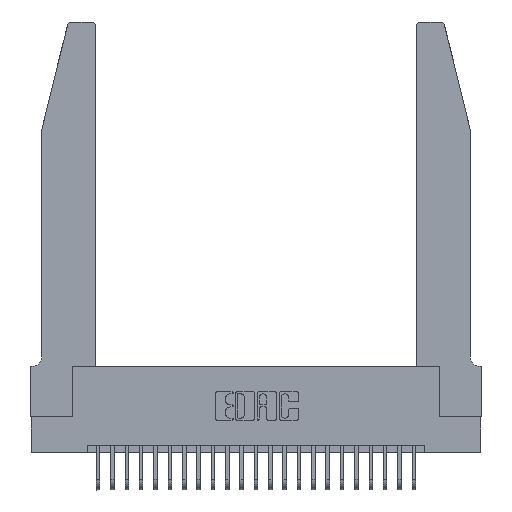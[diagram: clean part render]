
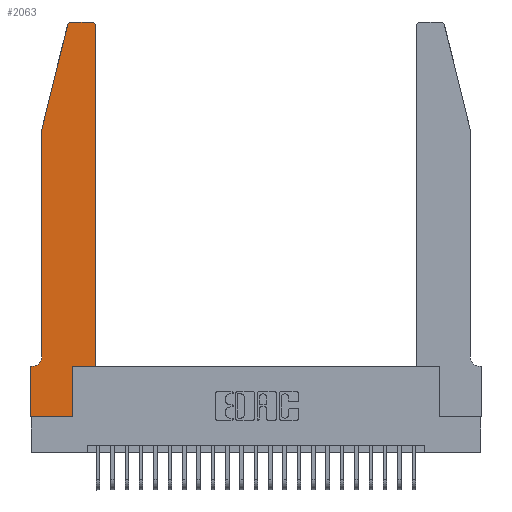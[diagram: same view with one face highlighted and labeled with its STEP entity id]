
A CAD part, top view. The second image highlights one B-rep face of the part: STEP entity #2063.
In plain terms, the highlighted planar face has unit normal (0, 0, 1).
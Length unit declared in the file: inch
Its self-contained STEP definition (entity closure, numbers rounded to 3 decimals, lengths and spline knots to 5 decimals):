
#255 = CARTESIAN_POINT ( 'NONE',  ( 0.0755, 2., 0.37 ) ) ;
#634 = CARTESIAN_POINT ( 'NONE',  ( 0., 0., 0.37 ) ) ;
#1424 = VERTEX_POINT ( 'NONE', #16039 ) ;
#1889 = EDGE_LOOP ( 'NONE', ( #6071, #23016, #17756, #4951, #12885, #19404, #13412, #17448, #3486, #7218, #13497, #17873 ) ) ;
#1991 = LINE ( 'NONE', #4695, #21640 ) ;
#2051 = VERTEX_POINT ( 'NONE', #19580 ) ;
#2063 = ADVANCED_FACE ( 'NONE', ( #15462 ), #19659, .T. ) ;
#2264 = EDGE_CURVE ( 'NONE', #1424, #14325, #13968, .T. ) ;
#2562 = VECTOR ( 'NONE', #20747, 39.37008 ) ;
#2923 = CARTESIAN_POINT ( 'NONE',  ( 0.4505, 0.35, 0.37 ) ) ;
#3486 = ORIENTED_EDGE ( 'NONE', *, *, #2264, .T. ) ;
#3692 = VERTEX_POINT ( 'NONE', #4216 ) ;
#3721 = VERTEX_POINT ( 'NONE', #19415 ) ;
#4216 = CARTESIAN_POINT ( 'NONE',  ( 0., 0.35, 0.37 ) ) ;
#4343 = VECTOR ( 'NONE', #16504, 39.37008 ) ;
#4695 = CARTESIAN_POINT ( 'NONE',  ( 0.0755, 0.35, 0.37 ) ) ;
#4836 = CARTESIAN_POINT ( 'NONE',  ( 0.0755, 2., 0.37 ) ) ;
#4951 = ORIENTED_EDGE ( 'NONE', *, *, #17871, .T. ) ;
#4970 = CARTESIAN_POINT ( 'NONE',  ( 0.4505, 0.35, 0.37 ) ) ;
#5073 = CARTESIAN_POINT ( 'NONE',  ( 0.2865, 0.35, 0.37 ) ) ;
#5242 = DIRECTION ( 'NONE',  ( 0., 0., 1. ) ) ;
#5247 = EDGE_CURVE ( 'NONE', #5578, #20814, #10075, .T. ) ;
#5578 = VERTEX_POINT ( 'NONE', #21055 ) ;
#6071 = ORIENTED_EDGE ( 'NONE', *, *, #19538, .T. ) ;
#6545 = CARTESIAN_POINT ( 'NONE',  ( 0.284, 2.72, 0.37 ) ) ;
#6816 = EDGE_CURVE ( 'NONE', #21677, #11515, #20289, .T. ) ;
#6902 = EDGE_CURVE ( 'NONE', #15831, #1424, #8905, .T. ) ;
#7218 = ORIENTED_EDGE ( 'NONE', *, *, #23342, .T. ) ;
#7433 = CARTESIAN_POINT ( 'NONE',  ( 0.2865, 0.35, 0.37 ) ) ;
#7582 = DIRECTION ( 'NONE',  ( 0., 0., -1. ) ) ;
#7660 = VERTEX_POINT ( 'NONE', #18802 ) ;
#8423 = CARTESIAN_POINT ( 'NONE',  ( 0., 0.35, 0.37 ) ) ;
#8494 = DIRECTION ( 'NONE',  ( 1., 0., 0. ) ) ;
#8838 = CARTESIAN_POINT ( 'NONE',  ( 0.2605, 2.75, 0.37 ) ) ;
#8905 = LINE ( 'NONE', #18409, #18271 ) ;
#9474 = VECTOR ( 'NONE', #10660, 39.37008 ) ;
#9624 = CARTESIAN_POINT ( 'NONE',  ( 0.284, 2.75, 0.37 ) ) ;
#9784 = CIRCLE ( 'NONE', #14880, 0.03 ) ;
#10075 = LINE ( 'NONE', #4836, #9474 ) ;
#10392 = VECTOR ( 'NONE', #14534, 39.37008 ) ;
#10399 = DIRECTION ( 'NONE',  ( 1., 0., 0. ) ) ;
#10660 = DIRECTION ( 'NONE',  ( -0.239, -0.971, 0. ) ) ;
#11042 = CARTESIAN_POINT ( 'NONE',  ( 0.0755, 2., 0.37 ) ) ;
#11326 = AXIS2_PLACEMENT_3D ( 'NONE', #6545, #19733, #8494 ) ;
#11515 = VERTEX_POINT ( 'NONE', #20967 ) ;
#12885 = ORIENTED_EDGE ( 'NONE', *, *, #17505, .T. ) ;
#13412 = ORIENTED_EDGE ( 'NONE', *, *, #21923, .T. ) ;
#13497 = ORIENTED_EDGE ( 'NONE', *, *, #6816, .T. ) ;
#13968 = LINE ( 'NONE', #5073, #4343 ) ;
#14325 = VERTEX_POINT ( 'NONE', #7433 ) ;
#14358 = DIRECTION ( 'NONE',  ( -1., 0., 0. ) ) ;
#14534 = DIRECTION ( 'NONE',  ( 0., 1., 0. ) ) ;
#14780 = DIRECTION ( 'NONE',  ( 0., -1., 0. ) ) ;
#14880 = AXIS2_PLACEMENT_3D ( 'NONE', #16644, #5242, #18508 ) ;
#15425 = CARTESIAN_POINT ( 'NONE',  ( 0., 0., 0.37 ) ) ;
#15439 = LINE ( 'NONE', #11042, #19782 ) ;
#15462 = FACE_OUTER_BOUND ( 'NONE', #1889, .T. ) ;
#15831 = VERTEX_POINT ( 'NONE', #634 ) ;
#16039 = CARTESIAN_POINT ( 'NONE',  ( 0.2865, 0., 0.37 ) ) ;
#16504 = DIRECTION ( 'NONE',  ( 0., 1., 0. ) ) ;
#16644 = CARTESIAN_POINT ( 'NONE',  ( 0.4205, 2.72, 0.37 ) ) ;
#16955 = AXIS2_PLACEMENT_3D ( 'NONE', #8423, #21542, #10399 ) ;
#17030 = VECTOR ( 'NONE', #17295, 39.37008 ) ;
#17295 = DIRECTION ( 'NONE',  ( 0., -1., 0. ) ) ;
#17448 = ORIENTED_EDGE ( 'NONE', *, *, #6902, .T. ) ;
#17505 = EDGE_CURVE ( 'NONE', #7660, #3721, #18050, .T. ) ;
#17756 = ORIENTED_EDGE ( 'NONE', *, *, #5247, .T. ) ;
#17871 = EDGE_CURVE ( 'NONE', #20814, #7660, #15439, .T. ) ;
#17873 = ORIENTED_EDGE ( 'NONE', *, *, #19961, .T. ) ;
#18050 = CIRCLE ( 'NONE', #22010, 0.07 ) ;
#18271 = VECTOR ( 'NONE', #20378, 39.37008 ) ;
#18376 = LINE ( 'NONE', #18868, #2562 ) ;
#18409 = CARTESIAN_POINT ( 'NONE',  ( 0., 0., 0.37 ) ) ;
#18508 = DIRECTION ( 'NONE',  ( 1., 0., 0. ) ) ;
#18802 = CARTESIAN_POINT ( 'NONE',  ( 0.0755, 0.42, 0.37 ) ) ;
#18848 = CARTESIAN_POINT ( 'NONE',  ( 0.0055, 0.42, 0.37 ) ) ;
#18868 = CARTESIAN_POINT ( 'NONE',  ( 0.4505, 0.35, 0.37 ) ) ;
#19129 = LINE ( 'NONE', #8838, #23526 ) ;
#19404 = ORIENTED_EDGE ( 'NONE', *, *, #22526, .T. ) ;
#19415 = CARTESIAN_POINT ( 'NONE',  ( 0.0055, 0.35, 0.37 ) ) ;
#19538 = EDGE_CURVE ( 'NONE', #2051, #23990, #19129, .T. ) ;
#19580 = CARTESIAN_POINT ( 'NONE',  ( 0.4205, 2.75, 0.37 ) ) ;
#19638 = CIRCLE ( 'NONE', #11326, 0.03 ) ;
#19659 = PLANE ( 'NONE',  #16955 ) ;
#19733 = DIRECTION ( 'NONE',  ( 0., 0., 1. ) ) ;
#19782 = VECTOR ( 'NONE', #14780, 39.37008 ) ;
#19961 = EDGE_CURVE ( 'NONE', #11515, #2051, #9784, .T. ) ;
#20289 = LINE ( 'NONE', #4970, #10392 ) ;
#20378 = DIRECTION ( 'NONE',  ( 1., 0., 0. ) ) ;
#20728 = DIRECTION ( 'NONE',  ( -1., 0., 0. ) ) ;
#20747 = DIRECTION ( 'NONE',  ( 1., 0., 0. ) ) ;
#20814 = VERTEX_POINT ( 'NONE', #255 ) ;
#20967 = CARTESIAN_POINT ( 'NONE',  ( 0.4505, 2.72, 0.37 ) ) ;
#21055 = CARTESIAN_POINT ( 'NONE',  ( 0.25487, 2.72718, 0.37 ) ) ;
#21533 = EDGE_CURVE ( 'NONE', #23990, #5578, #19638, .T. ) ;
#21542 = DIRECTION ( 'NONE',  ( 0., 0., 1. ) ) ;
#21640 = VECTOR ( 'NONE', #14358, 39.37008 ) ;
#21677 = VERTEX_POINT ( 'NONE', #2923 ) ;
#21923 = EDGE_CURVE ( 'NONE', #3692, #15831, #21986, .T. ) ;
#21944 = DIRECTION ( 'NONE',  ( -1., 0., 0. ) ) ;
#21986 = LINE ( 'NONE', #15425, #17030 ) ;
#22010 = AXIS2_PLACEMENT_3D ( 'NONE', #18848, #7582, #20728 ) ;
#22526 = EDGE_CURVE ( 'NONE', #3721, #3692, #1991, .T. ) ;
#23016 = ORIENTED_EDGE ( 'NONE', *, *, #21533, .T. ) ;
#23342 = EDGE_CURVE ( 'NONE', #14325, #21677, #18376, .T. ) ;
#23526 = VECTOR ( 'NONE', #21944, 39.37008 ) ;
#23990 = VERTEX_POINT ( 'NONE', #9624 ) ;
